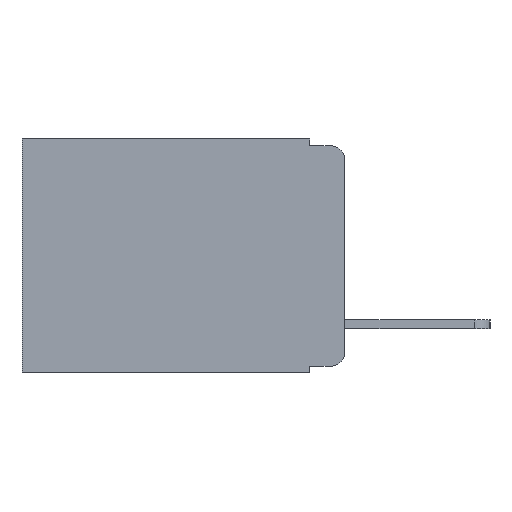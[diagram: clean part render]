
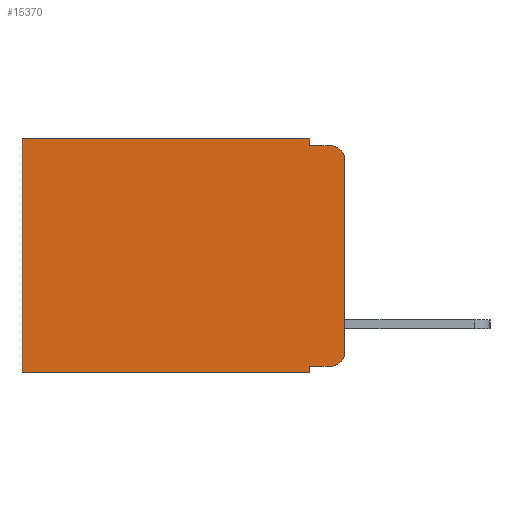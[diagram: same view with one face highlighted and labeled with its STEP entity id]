
A CAD part, left-side view. The second image highlights one B-rep face of the part: STEP entity #15370.
In plain terms, the highlighted planar face has unit normal (-1, 0, 0).
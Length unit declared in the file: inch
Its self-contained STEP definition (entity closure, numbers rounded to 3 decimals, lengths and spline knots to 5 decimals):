
#379 = LINE ( 'NONE', #14721, #15777 ) ;
#547 = EDGE_CURVE ( 'NONE', #14833, #18110, #18047, .T. ) ;
#1257 = VERTEX_POINT ( 'NONE', #10213 ) ;
#1364 = ORIENTED_EDGE ( 'NONE', *, *, #9729, .F. ) ;
#1477 = DIRECTION ( 'NONE',  ( 0., 0., -1. ) ) ;
#1531 = CARTESIAN_POINT ( 'NONE',  ( 0.298, 0., 0. ) ) ;
#1747 = EDGE_CURVE ( 'NONE', #18110, #8552, #18256, .T. ) ;
#1801 = DIRECTION ( 'NONE',  ( -1., 0., 0. ) ) ;
#2196 = CIRCLE ( 'NONE', #14501, 0.02 ) ;
#2210 = CARTESIAN_POINT ( 'NONE',  ( 0.298, 0.473, 0. ) ) ;
#2511 = EDGE_LOOP ( 'NONE', ( #1364, #16026, #14257, #3009, #9664, #4901, #2695, #4624, #5539, #13424 ) ) ;
#2695 = ORIENTED_EDGE ( 'NONE', *, *, #1747, .F. ) ;
#3009 = ORIENTED_EDGE ( 'NONE', *, *, #11566, .F. ) ;
#3711 = VERTEX_POINT ( 'NONE', #18292 ) ;
#3766 = VERTEX_POINT ( 'NONE', #17567 ) ;
#4262 = VECTOR ( 'NONE', #15267, 39.37008 ) ;
#4467 = VECTOR ( 'NONE', #13957, 39.37008 ) ;
#4534 = AXIS2_PLACEMENT_3D ( 'NONE', #15766, #12659, #18745 ) ;
#4624 = ORIENTED_EDGE ( 'NONE', *, *, #547, .F. ) ;
#4692 = DIRECTION ( 'NONE',  ( -1., 0., 0. ) ) ;
#4901 = ORIENTED_EDGE ( 'NONE', *, *, #11790, .T. ) ;
#4977 = DIRECTION ( 'NONE',  ( 0., 0., -1. ) ) ;
#5003 = DIRECTION ( 'NONE',  ( 0., 1., 0. ) ) ;
#5303 = LINE ( 'NONE', #18053, #8746 ) ;
#5460 = CARTESIAN_POINT ( 'NONE',  ( 0.298, 0., -0.343 ) ) ;
#5539 = ORIENTED_EDGE ( 'NONE', *, *, #7776, .T. ) ;
#5864 = DIRECTION ( 'NONE',  ( 0., 0., -1. ) ) ;
#6089 = VECTOR ( 'NONE', #5003, 39.37008 ) ;
#6598 = CARTESIAN_POINT ( 'NONE',  ( 0.298, 0.051, -0.01 ) ) ;
#7776 = EDGE_CURVE ( 'NONE', #14833, #10911, #8175, .T. ) ;
#8045 = DIRECTION ( 'NONE',  ( 0., -1., 0. ) ) ;
#8118 = EDGE_CURVE ( 'NONE', #17503, #9483, #14193, .T. ) ;
#8175 = LINE ( 'NONE', #17324, #4262 ) ;
#8516 = DIRECTION ( 'NONE',  ( 0., 1., 0. ) ) ;
#8552 = VERTEX_POINT ( 'NONE', #16645 ) ;
#8746 = VECTOR ( 'NONE', #4977, 39.37008 ) ;
#9483 = VERTEX_POINT ( 'NONE', #2210 ) ;
#9648 = CIRCLE ( 'NONE', #14366, 0.02 ) ;
#9664 = ORIENTED_EDGE ( 'NONE', *, *, #8118, .T. ) ;
#9729 = EDGE_CURVE ( 'NONE', #3711, #11410, #11998, .T. ) ;
#9782 = VECTOR ( 'NONE', #5864, 39.37008 ) ;
#10094 = CARTESIAN_POINT ( 'NONE',  ( 0.298, 0., -0.313 ) ) ;
#10213 = CARTESIAN_POINT ( 'NONE',  ( 0.298, 0.051, -0.01 ) ) ;
#10571 = CARTESIAN_POINT ( 'NONE',  ( 0.298, 0.051, 0. ) ) ;
#10607 = CARTESIAN_POINT ( 'NONE',  ( 0.298, 0.02, -0.313 ) ) ;
#10911 = VERTEX_POINT ( 'NONE', #18011 ) ;
#10987 = EDGE_CURVE ( 'NONE', #1257, #3766, #17216, .T. ) ;
#11410 = VERTEX_POINT ( 'NONE', #10094 ) ;
#11566 = EDGE_CURVE ( 'NONE', #17503, #1257, #379, .T. ) ;
#11790 = EDGE_CURVE ( 'NONE', #9483, #8552, #5303, .T. ) ;
#11987 = DIRECTION ( 'NONE',  ( 0., 0., -1. ) ) ;
#11998 = LINE ( 'NONE', #13503, #4467 ) ;
#12659 = DIRECTION ( 'NONE',  ( 1., 0., 0. ) ) ;
#12662 = VECTOR ( 'NONE', #8045, 39.37008 ) ;
#13275 = CARTESIAN_POINT ( 'NONE',  ( 0.298, 0.02, -0.03 ) ) ;
#13306 = CARTESIAN_POINT ( 'NONE',  ( 0.298, 0.051, -0.343 ) ) ;
#13424 = ORIENTED_EDGE ( 'NONE', *, *, #17528, .T. ) ;
#13503 = CARTESIAN_POINT ( 'NONE',  ( 0.298, 0., 0. ) ) ;
#13957 = DIRECTION ( 'NONE',  ( 0., 0., -1. ) ) ;
#13980 = CARTESIAN_POINT ( 'NONE',  ( 0.298, 0.051, -0.333 ) ) ;
#14193 = LINE ( 'NONE', #1531, #6089 ) ;
#14257 = ORIENTED_EDGE ( 'NONE', *, *, #10987, .F. ) ;
#14366 = AXIS2_PLACEMENT_3D ( 'NONE', #13275, #4692, #14821 ) ;
#14501 = AXIS2_PLACEMENT_3D ( 'NONE', #10607, #1801, #11987 ) ;
#14721 = CARTESIAN_POINT ( 'NONE',  ( 0.298, 0.051, 0. ) ) ;
#14821 = DIRECTION ( 'NONE',  ( 0., 0., -1. ) ) ;
#14833 = VERTEX_POINT ( 'NONE', #13980 ) ;
#15267 = DIRECTION ( 'NONE',  ( 0., -1., 0. ) ) ;
#15370 = ADVANCED_FACE ( 'NONE', ( #15382 ), #17279, .F. ) ;
#15382 = FACE_OUTER_BOUND ( 'NONE', #2511, .T. ) ;
#15766 = CARTESIAN_POINT ( 'NONE',  ( 0.298, 0., 0. ) ) ;
#15777 = VECTOR ( 'NONE', #1477, 39.37008 ) ;
#16026 = ORIENTED_EDGE ( 'NONE', *, *, #16365, .T. ) ;
#16365 = EDGE_CURVE ( 'NONE', #3711, #3766, #9648, .T. ) ;
#16391 = CARTESIAN_POINT ( 'NONE',  ( 0.298, 0.051, 0. ) ) ;
#16645 = CARTESIAN_POINT ( 'NONE',  ( 0.298, 0.473, -0.343 ) ) ;
#17216 = LINE ( 'NONE', #6598, #12662 ) ;
#17279 = PLANE ( 'NONE',  #4534 ) ;
#17324 = CARTESIAN_POINT ( 'NONE',  ( 0.298, 0.051, -0.333 ) ) ;
#17503 = VERTEX_POINT ( 'NONE', #16391 ) ;
#17528 = EDGE_CURVE ( 'NONE', #10911, #11410, #2196, .T. ) ;
#17567 = CARTESIAN_POINT ( 'NONE',  ( 0.298, 0.02, -0.01 ) ) ;
#18011 = CARTESIAN_POINT ( 'NONE',  ( 0.298, 0.02, -0.333 ) ) ;
#18047 = LINE ( 'NONE', #10571, #9782 ) ;
#18053 = CARTESIAN_POINT ( 'NONE',  ( 0.298, 0.473, 0. ) ) ;
#18110 = VERTEX_POINT ( 'NONE', #13306 ) ;
#18256 = LINE ( 'NONE', #5460, #19180 ) ;
#18292 = CARTESIAN_POINT ( 'NONE',  ( 0.298, 0., -0.03 ) ) ;
#18745 = DIRECTION ( 'NONE',  ( 0., 0., -1. ) ) ;
#19180 = VECTOR ( 'NONE', #8516, 39.37008 ) ;
